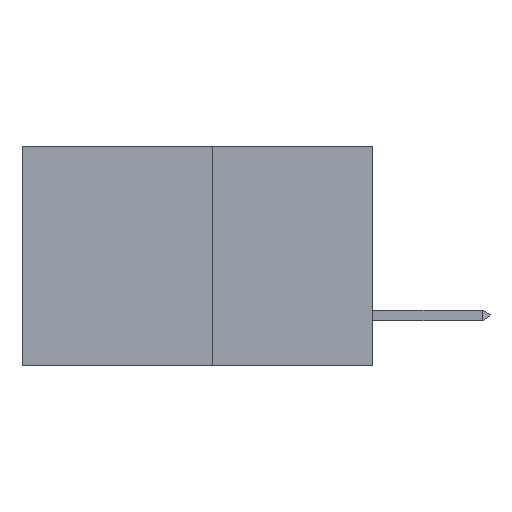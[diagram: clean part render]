
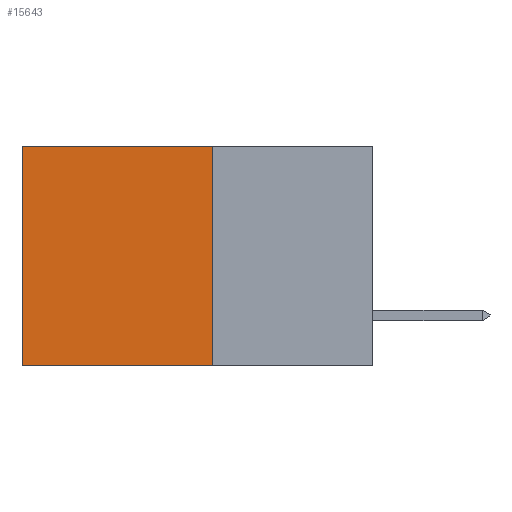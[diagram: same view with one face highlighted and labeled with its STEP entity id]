
A CAD part, left-side view. The second image highlights one B-rep face of the part: STEP entity #15643.
In plain terms, the highlighted planar face has unit normal (-1, 0, 0).
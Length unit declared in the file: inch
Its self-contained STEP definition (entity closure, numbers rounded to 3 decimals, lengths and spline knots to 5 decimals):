
#1086 = DIRECTION ( 'NONE',  ( 0., 1., 0. ) ) ;
#1291 = VECTOR ( 'NONE', #1086, 39.37008 ) ;
#2594 = EDGE_LOOP ( 'NONE', ( #10735, #5902, #8742, #18715 ) ) ;
#2894 = VERTEX_POINT ( 'NONE', #5299 ) ;
#2974 = EDGE_CURVE ( 'NONE', #2894, #5685, #20995, .T. ) ;
#3063 = CARTESIAN_POINT ( 'NONE',  ( 0.277, 0.59, -0.37 ) ) ;
#4483 = CARTESIAN_POINT ( 'NONE',  ( 0.277, 0.27, -0.37 ) ) ;
#4543 = CARTESIAN_POINT ( 'NONE',  ( 0.277, 0.27, 0. ) ) ;
#4729 = CARTESIAN_POINT ( 'NONE',  ( 0.277, 0.59, -0.37 ) ) ;
#5299 = CARTESIAN_POINT ( 'NONE',  ( 0.277, 0.59, 0. ) ) ;
#5685 = VERTEX_POINT ( 'NONE', #3063 ) ;
#5713 = DIRECTION ( 'NONE',  ( 0., 0., -1. ) ) ;
#5902 = ORIENTED_EDGE ( 'NONE', *, *, #14507, .F. ) ;
#6087 = VECTOR ( 'NONE', #8499, 39.37008 ) ;
#6745 = CARTESIAN_POINT ( 'NONE',  ( 0.277, 0.27, -0.37 ) ) ;
#7995 = PLANE ( 'NONE',  #14671 ) ;
#8499 = DIRECTION ( 'NONE',  ( 0., 1., 0. ) ) ;
#8742 = ORIENTED_EDGE ( 'NONE', *, *, #21472, .F. ) ;
#9764 = DIRECTION ( 'NONE',  ( 0., 0., -1. ) ) ;
#9819 = VERTEX_POINT ( 'NONE', #14830 ) ;
#10735 = ORIENTED_EDGE ( 'NONE', *, *, #2974, .T. ) ;
#10817 = LINE ( 'NONE', #14383, #14881 ) ;
#11143 = LINE ( 'NONE', #4543, #1291 ) ;
#12389 = CARTESIAN_POINT ( 'NONE',  ( 0.277, 0.27, -0.37 ) ) ;
#14383 = CARTESIAN_POINT ( 'NONE',  ( 0.277, 0.27, -0.37 ) ) ;
#14507 = EDGE_CURVE ( 'NONE', #22523, #5685, #19954, .T. ) ;
#14671 = AXIS2_PLACEMENT_3D ( 'NONE', #4483, #20133, #9764 ) ;
#14830 = CARTESIAN_POINT ( 'NONE',  ( 0.277, 0.27, 0. ) ) ;
#14881 = VECTOR ( 'NONE', #5713, 39.37008 ) ;
#15643 = ADVANCED_FACE ( 'NONE', ( #19077 ), #7995, .F. ) ;
#17240 = DIRECTION ( 'NONE',  ( 0., 0., -1. ) ) ;
#18715 = ORIENTED_EDGE ( 'NONE', *, *, #20425, .T. ) ;
#19077 = FACE_OUTER_BOUND ( 'NONE', #2594, .T. ) ;
#19954 = LINE ( 'NONE', #6745, #6087 ) ;
#20133 = DIRECTION ( 'NONE',  ( 1., 0., 0. ) ) ;
#20425 = EDGE_CURVE ( 'NONE', #9819, #2894, #11143, .T. ) ;
#20995 = LINE ( 'NONE', #4729, #21534 ) ;
#21472 = EDGE_CURVE ( 'NONE', #9819, #22523, #10817, .T. ) ;
#21534 = VECTOR ( 'NONE', #17240, 39.37008 ) ;
#22523 = VERTEX_POINT ( 'NONE', #12389 ) ;
